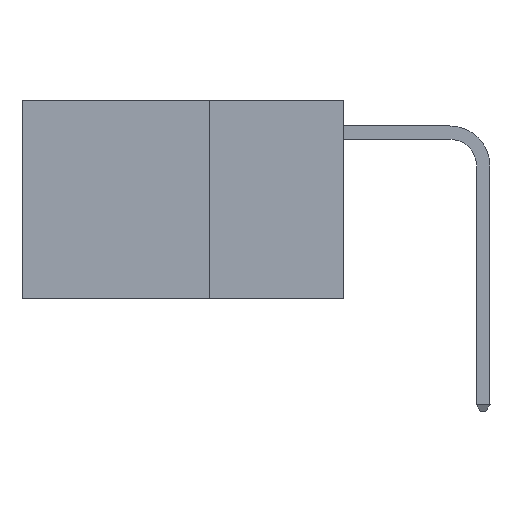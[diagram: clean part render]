
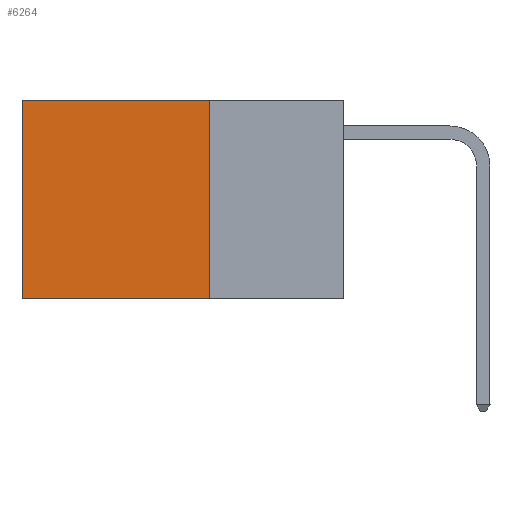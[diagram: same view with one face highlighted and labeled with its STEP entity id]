
A CAD part, left-side view. The second image highlights one B-rep face of the part: STEP entity #6264.
In plain terms, the highlighted planar face has unit normal (-1, 0, 0).
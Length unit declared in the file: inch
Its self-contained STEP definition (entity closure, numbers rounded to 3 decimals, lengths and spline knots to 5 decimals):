
#1572 = EDGE_CURVE ( 'NONE', #20856, #10646, #9745, .T. ) ;
#1804 = EDGE_CURVE ( 'NONE', #13713, #12264, #9310, .T. ) ;
#3814 = CARTESIAN_POINT ( 'NONE',  ( 0.2625, 0.25, 0. ) ) ;
#4069 = LINE ( 'NONE', #7778, #9791 ) ;
#4164 = DIRECTION ( 'NONE',  ( 0., 1., 0. ) ) ;
#5042 = CARTESIAN_POINT ( 'NONE',  ( 0.2625, 0.6, 0. ) ) ;
#5229 = CARTESIAN_POINT ( 'NONE',  ( 0.2625, 0.6, 0. ) ) ;
#5488 = LINE ( 'NONE', #5229, #12467 ) ;
#5669 = DIRECTION ( 'NONE',  ( 0., 0., -1. ) ) ;
#5672 = DIRECTION ( 'NONE',  ( 1., 0., 0. ) ) ;
#6264 = ADVANCED_FACE ( 'NONE', ( #11738 ), #25741, .F. ) ;
#7567 = AXIS2_PLACEMENT_3D ( 'NONE', #3814, #5672, #9369 ) ;
#7778 = CARTESIAN_POINT ( 'NONE',  ( 0.2625, 0.25, 0. ) ) ;
#9310 = LINE ( 'NONE', #19103, #15745 ) ;
#9369 = DIRECTION ( 'NONE',  ( 0., 0., -1. ) ) ;
#9604 = ORIENTED_EDGE ( 'NONE', *, *, #1804, .T. ) ;
#9745 = LINE ( 'NONE', #22154, #24183 ) ;
#9791 = VECTOR ( 'NONE', #5669, 39.37008 ) ;
#10646 = VERTEX_POINT ( 'NONE', #18788 ) ;
#10909 = DIRECTION ( 'NONE',  ( 0., 0., -1. ) ) ;
#11563 = DIRECTION ( 'NONE',  ( 0., 1., 0. ) ) ;
#11738 = FACE_OUTER_BOUND ( 'NONE', #12158, .T. ) ;
#12158 = EDGE_LOOP ( 'NONE', ( #21393, #19817, #22396, #9604 ) ) ;
#12264 = VERTEX_POINT ( 'NONE', #5042 ) ;
#12467 = VECTOR ( 'NONE', #10909, 39.37008 ) ;
#12960 = CARTESIAN_POINT ( 'NONE',  ( 0.2625, 0.25, -0.37 ) ) ;
#13713 = VERTEX_POINT ( 'NONE', #13833 ) ;
#13833 = CARTESIAN_POINT ( 'NONE',  ( 0.2625, 0.25, 0. ) ) ;
#13995 = EDGE_CURVE ( 'NONE', #12264, #10646, #5488, .T. ) ;
#15745 = VECTOR ( 'NONE', #11563, 39.37008 ) ;
#18788 = CARTESIAN_POINT ( 'NONE',  ( 0.2625, 0.6, -0.37 ) ) ;
#19103 = CARTESIAN_POINT ( 'NONE',  ( 0.2625, 0.25, 0. ) ) ;
#19817 = ORIENTED_EDGE ( 'NONE', *, *, #1572, .F. ) ;
#20856 = VERTEX_POINT ( 'NONE', #12960 ) ;
#21393 = ORIENTED_EDGE ( 'NONE', *, *, #13995, .T. ) ;
#22154 = CARTESIAN_POINT ( 'NONE',  ( 0.2625, 0.25, -0.37 ) ) ;
#22396 = ORIENTED_EDGE ( 'NONE', *, *, #24766, .F. ) ;
#24183 = VECTOR ( 'NONE', #4164, 39.37008 ) ;
#24766 = EDGE_CURVE ( 'NONE', #13713, #20856, #4069, .T. ) ;
#25741 = PLANE ( 'NONE',  #7567 ) ;
